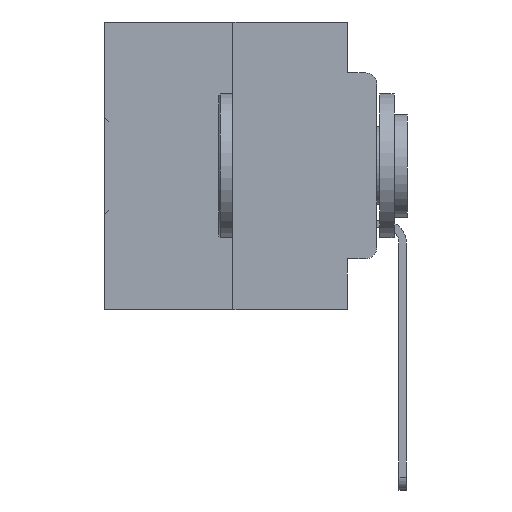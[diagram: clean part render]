
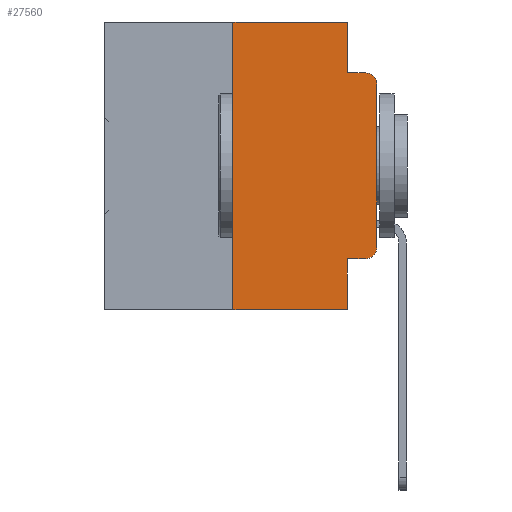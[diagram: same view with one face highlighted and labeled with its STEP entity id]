
A CAD part, left-side view. The second image highlights one B-rep face of the part: STEP entity #27560.
In plain terms, the highlighted planar face has unit normal (-1, 0, 0).
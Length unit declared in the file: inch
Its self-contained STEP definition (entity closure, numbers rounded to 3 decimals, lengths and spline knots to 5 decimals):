
#677 = ORIENTED_EDGE ( 'NONE', *, *, #811, .F. ) ;
#811 = EDGE_CURVE ( 'NONE', #22326, #9790, #7129, .T. ) ;
#988 = CARTESIAN_POINT ( 'NONE',  ( 0., 0.051, 0. ) ) ;
#1443 = CARTESIAN_POINT ( 'NONE',  ( 0., 0.25, 0. ) ) ;
#2113 = ORIENTED_EDGE ( 'NONE', *, *, #5548, .F. ) ;
#2135 = VERTEX_POINT ( 'NONE', #988 ) ;
#2211 = LINE ( 'NONE', #8541, #8645 ) ;
#3569 = FACE_OUTER_BOUND ( 'NONE', #7460, .T. ) ;
#3955 = LINE ( 'NONE', #34875, #33372 ) ;
#4417 = LINE ( 'NONE', #24383, #24695 ) ;
#4686 = DIRECTION ( 'NONE',  ( 0., -1., 0. ) ) ;
#4961 = VECTOR ( 'NONE', #5215, 39.37008 ) ;
#5127 = EDGE_CURVE ( 'NONE', #22326, #27807, #17977, .T. ) ;
#5215 = DIRECTION ( 'NONE',  ( 0., -1., 0. ) ) ;
#5548 = EDGE_CURVE ( 'NONE', #9031, #18632, #32543, .T. ) ;
#6242 = CARTESIAN_POINT ( 'NONE',  ( 0., 0.02, -0.1085 ) ) ;
#6399 = CARTESIAN_POINT ( 'NONE',  ( 0., 0.473, 0. ) ) ;
#7028 = LINE ( 'NONE', #16950, #35403 ) ;
#7129 = LINE ( 'NONE', #15186, #20065 ) ;
#7252 = EDGE_CURVE ( 'NONE', #35496, #9790, #3955, .T. ) ;
#7363 = CARTESIAN_POINT ( 'NONE',  ( 0., 0.02, -0.0885 ) ) ;
#7460 = EDGE_LOOP ( 'NONE', ( #31591, #31627, #2113, #15560, #32751, #11311, #18641, #677, #13247, #21848 ) ) ;
#8163 = EDGE_CURVE ( 'NONE', #35496, #10349, #19939, .T. ) ;
#8541 = CARTESIAN_POINT ( 'NONE',  ( 0., 0.473, 0. ) ) ;
#8645 = VECTOR ( 'NONE', #11370, 39.37008 ) ;
#9023 = DIRECTION ( 'NONE',  ( 0., 0., -1. ) ) ;
#9031 = VERTEX_POINT ( 'NONE', #14935 ) ;
#9172 = DIRECTION ( 'NONE',  ( 1., 0., 0. ) ) ;
#9790 = VERTEX_POINT ( 'NONE', #10039 ) ;
#10039 = CARTESIAN_POINT ( 'NONE',  ( 0., 0.051, -0.5 ) ) ;
#10349 = VERTEX_POINT ( 'NONE', #1443 ) ;
#11311 = ORIENTED_EDGE ( 'NONE', *, *, #8163, .F. ) ;
#11370 = DIRECTION ( 'NONE',  ( 0., -1., 0. ) ) ;
#12003 = CARTESIAN_POINT ( 'NONE',  ( 0., 0.051, -0.4115 ) ) ;
#12670 = VECTOR ( 'NONE', #13855, 39.37008 ) ;
#13247 = ORIENTED_EDGE ( 'NONE', *, *, #5127, .T. ) ;
#13665 = AXIS2_PLACEMENT_3D ( 'NONE', #6242, #25515, #9023 ) ;
#13801 = CARTESIAN_POINT ( 'NONE',  ( 0., 0.25, -0.5 ) ) ;
#13855 = DIRECTION ( 'NONE',  ( 0., 0., 1. ) ) ;
#14401 = DIRECTION ( 'NONE',  ( -1., 0., 0. ) ) ;
#14679 = CARTESIAN_POINT ( 'NONE',  ( 0., 0., -0.1085 ) ) ;
#14935 = CARTESIAN_POINT ( 'NONE',  ( 0., 0.051, -0.0885 ) ) ;
#15186 = CARTESIAN_POINT ( 'NONE',  ( 0., 0.051, 0. ) ) ;
#15533 = EDGE_CURVE ( 'NONE', #10349, #2135, #2211, .T. ) ;
#15560 = ORIENTED_EDGE ( 'NONE', *, *, #34851, .F. ) ;
#16950 = CARTESIAN_POINT ( 'NONE',  ( 0., 0., 0. ) ) ;
#17128 = VECTOR ( 'NONE', #31123, 39.37008 ) ;
#17977 = LINE ( 'NONE', #22867, #17128 ) ;
#18632 = VERTEX_POINT ( 'NONE', #7363 ) ;
#18641 = ORIENTED_EDGE ( 'NONE', *, *, #7252, .T. ) ;
#19939 = LINE ( 'NONE', #33034, #12670 ) ;
#20065 = VECTOR ( 'NONE', #35512, 39.37008 ) ;
#21848 = ORIENTED_EDGE ( 'NONE', *, *, #25658, .T. ) ;
#22326 = VERTEX_POINT ( 'NONE', #12003 ) ;
#22456 = VERTEX_POINT ( 'NONE', #34528 ) ;
#22867 = CARTESIAN_POINT ( 'NONE',  ( 0., 0.051, -0.4115 ) ) ;
#22923 = PLANE ( 'NONE',  #29634 ) ;
#23553 = AXIS2_PLACEMENT_3D ( 'NONE', #30830, #14401, #33585 ) ;
#23979 = VERTEX_POINT ( 'NONE', #14679 ) ;
#24383 = CARTESIAN_POINT ( 'NONE',  ( 0., 0.051, 0. ) ) ;
#24695 = VECTOR ( 'NONE', #35272, 39.37008 ) ;
#25515 = DIRECTION ( 'NONE',  ( -1., 0., 0. ) ) ;
#25658 = EDGE_CURVE ( 'NONE', #27807, #22456, #35529, .T. ) ;
#25713 = CIRCLE ( 'NONE', #13665, 0.02 ) ;
#26752 = CARTESIAN_POINT ( 'NONE',  ( 0., 0.02, -0.4115 ) ) ;
#27460 = EDGE_CURVE ( 'NONE', #22456, #23979, #7028, .T. ) ;
#27560 = ADVANCED_FACE ( 'NONE', ( #3569 ), #22923, .F. ) ;
#27807 = VERTEX_POINT ( 'NONE', #26752 ) ;
#27960 = DIRECTION ( 'NONE',  ( 0., 0., 1. ) ) ;
#28438 = DIRECTION ( 'NONE',  ( 0., 0., -1. ) ) ;
#29634 = AXIS2_PLACEMENT_3D ( 'NONE', #6399, #9172, #28438 ) ;
#30830 = CARTESIAN_POINT ( 'NONE',  ( 0., 0.02, -0.3915 ) ) ;
#31123 = DIRECTION ( 'NONE',  ( 0., -1., 0. ) ) ;
#31591 = ORIENTED_EDGE ( 'NONE', *, *, #27460, .T. ) ;
#31627 = ORIENTED_EDGE ( 'NONE', *, *, #32761, .T. ) ;
#32543 = LINE ( 'NONE', #32676, #4961 ) ;
#32676 = CARTESIAN_POINT ( 'NONE',  ( 0., 0.051, -0.0885 ) ) ;
#32751 = ORIENTED_EDGE ( 'NONE', *, *, #15533, .F. ) ;
#32761 = EDGE_CURVE ( 'NONE', #23979, #18632, #25713, .T. ) ;
#33034 = CARTESIAN_POINT ( 'NONE',  ( 0., 0.25, 0. ) ) ;
#33372 = VECTOR ( 'NONE', #4686, 39.37008 ) ;
#33585 = DIRECTION ( 'NONE',  ( 0., 0., -1. ) ) ;
#34528 = CARTESIAN_POINT ( 'NONE',  ( 0., 0., -0.3915 ) ) ;
#34851 = EDGE_CURVE ( 'NONE', #2135, #9031, #4417, .T. ) ;
#34875 = CARTESIAN_POINT ( 'NONE',  ( 0., 0.473, -0.5 ) ) ;
#35272 = DIRECTION ( 'NONE',  ( 0., 0., -1. ) ) ;
#35403 = VECTOR ( 'NONE', #27960, 39.37008 ) ;
#35496 = VERTEX_POINT ( 'NONE', #13801 ) ;
#35512 = DIRECTION ( 'NONE',  ( 0., 0., -1. ) ) ;
#35529 = CIRCLE ( 'NONE', #23553, 0.02 ) ;
